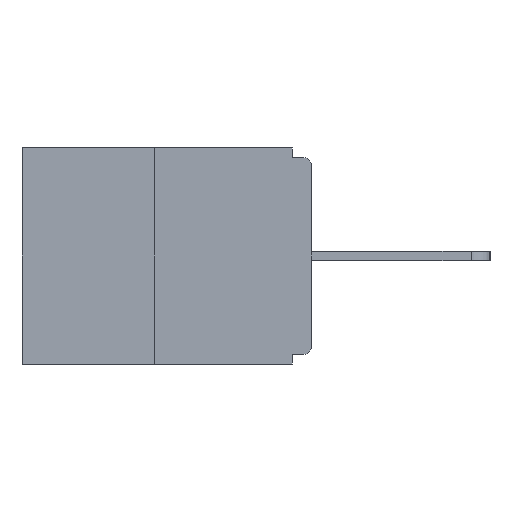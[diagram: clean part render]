
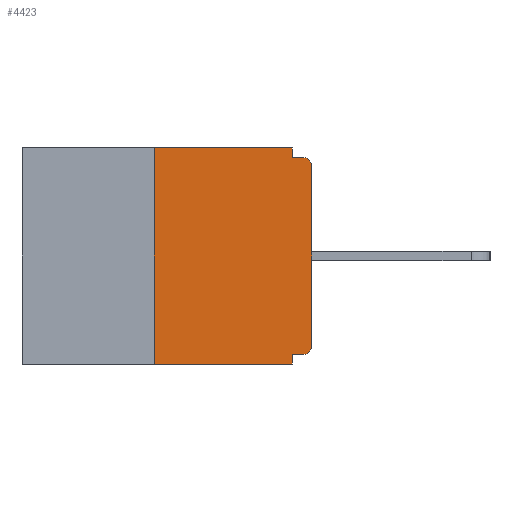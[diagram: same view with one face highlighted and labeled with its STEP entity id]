
A CAD part, left-side view. The second image highlights one B-rep face of the part: STEP entity #4423.
In plain terms, the highlighted planar face has unit normal (-1, 0, 0).
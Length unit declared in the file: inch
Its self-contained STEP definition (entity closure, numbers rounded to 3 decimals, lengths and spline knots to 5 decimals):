
#121 = VECTOR ( 'NONE', #13060, 39.37008 ) ;
#340 = DIRECTION ( 'NONE',  ( 0., -1., 0. ) ) ;
#589 = LINE ( 'NONE', #2105, #20550 ) ;
#617 = EDGE_CURVE ( 'NONE', #13745, #7215, #2869, .T. ) ;
#618 = ORIENTED_EDGE ( 'NONE', *, *, #7090, .F. ) ;
#761 = DIRECTION ( 'NONE',  ( 0., 0., -1. ) ) ;
#1275 = VECTOR ( 'NONE', #15294, 39.37008 ) ;
#1450 = CARTESIAN_POINT ( 'NONE',  ( 0., 0., -0.03 ) ) ;
#1510 = AXIS2_PLACEMENT_3D ( 'NONE', #13704, #17521, #15664 ) ;
#1878 = CARTESIAN_POINT ( 'NONE',  ( 0., 0.031, -0.015 ) ) ;
#2105 = CARTESIAN_POINT ( 'NONE',  ( 0., 0., -0.015 ) ) ;
#2442 = VERTEX_POINT ( 'NONE', #18229 ) ;
#2542 = ORIENTED_EDGE ( 'NONE', *, *, #14421, .F. ) ;
#2869 = CIRCLE ( 'NONE', #14694, 0.015 ) ;
#3036 = CARTESIAN_POINT ( 'NONE',  ( 0., 0., 0. ) ) ;
#3769 = CARTESIAN_POINT ( 'NONE',  ( 0., 0.46, 0. ) ) ;
#4001 = DIRECTION ( 'NONE',  ( 1., 0., 0. ) ) ;
#4075 = DIRECTION ( 'NONE',  ( 0., -1., 0. ) ) ;
#4110 = FACE_OUTER_BOUND ( 'NONE', #20853, .T. ) ;
#4326 = VERTEX_POINT ( 'NONE', #15697 ) ;
#4423 = ADVANCED_FACE ( 'NONE', ( #4110 ), #7456, .F. ) ;
#4606 = VERTEX_POINT ( 'NONE', #6181 ) ;
#5481 = DIRECTION ( 'NONE',  ( 0., 0., -1. ) ) ;
#5856 = ORIENTED_EDGE ( 'NONE', *, *, #6745, .F. ) ;
#5961 = CIRCLE ( 'NONE', #1510, 0.015 ) ;
#6181 = CARTESIAN_POINT ( 'NONE',  ( 0., 0.25, -0.343 ) ) ;
#6287 = EDGE_CURVE ( 'NONE', #17212, #13745, #14839, .T. ) ;
#6362 = ORIENTED_EDGE ( 'NONE', *, *, #16251, .T. ) ;
#6635 = ORIENTED_EDGE ( 'NONE', *, *, #20191, .F. ) ;
#6745 = EDGE_CURVE ( 'NONE', #4606, #4326, #9105, .T. ) ;
#6884 = AXIS2_PLACEMENT_3D ( 'NONE', #3769, #4001, #10833 ) ;
#7090 = EDGE_CURVE ( 'NONE', #10449, #21361, #14043, .T. ) ;
#7215 = VERTEX_POINT ( 'NONE', #16700 ) ;
#7456 = PLANE ( 'NONE',  #6884 ) ;
#8200 = LINE ( 'NONE', #15263, #121 ) ;
#8759 = DIRECTION ( 'NONE',  ( 0., 0., 1. ) ) ;
#9105 = LINE ( 'NONE', #19409, #10096 ) ;
#9154 = LINE ( 'NONE', #16207, #9978 ) ;
#9737 = LINE ( 'NONE', #20509, #1275 ) ;
#9885 = ORIENTED_EDGE ( 'NONE', *, *, #617, .T. ) ;
#9978 = VECTOR ( 'NONE', #340, 39.37008 ) ;
#10065 = VERTEX_POINT ( 'NONE', #20390 ) ;
#10096 = VECTOR ( 'NONE', #8759, 39.37008 ) ;
#10190 = EDGE_CURVE ( 'NONE', #17367, #10065, #9737, .T. ) ;
#10449 = VERTEX_POINT ( 'NONE', #19798 ) ;
#10833 = DIRECTION ( 'NONE',  ( 0., 0., -1. ) ) ;
#11376 = DIRECTION ( 'NONE',  ( 0., 0., 1. ) ) ;
#11889 = ORIENTED_EDGE ( 'NONE', *, *, #22378, .F. ) ;
#12240 = CARTESIAN_POINT ( 'NONE',  ( 0., 0., -0.313 ) ) ;
#12807 = ORIENTED_EDGE ( 'NONE', *, *, #6287, .T. ) ;
#13032 = CARTESIAN_POINT ( 'NONE',  ( 0., 0.015, -0.03 ) ) ;
#13060 = DIRECTION ( 'NONE',  ( 0., 0., -1. ) ) ;
#13455 = LINE ( 'NONE', #16692, #21918 ) ;
#13704 = CARTESIAN_POINT ( 'NONE',  ( 0., 0.015, -0.313 ) ) ;
#13745 = VERTEX_POINT ( 'NONE', #1450 ) ;
#14043 = LINE ( 'NONE', #22842, #20082 ) ;
#14129 = VECTOR ( 'NONE', #11376, 39.37008 ) ;
#14421 = EDGE_CURVE ( 'NONE', #4326, #10449, #9154, .T. ) ;
#14694 = AXIS2_PLACEMENT_3D ( 'NONE', #13032, #21727, #761 ) ;
#14839 = LINE ( 'NONE', #3036, #14129 ) ;
#14956 = DIRECTION ( 'NONE',  ( 0., -1., 0. ) ) ;
#15263 = CARTESIAN_POINT ( 'NONE',  ( 0., 0.031, -0.343 ) ) ;
#15294 = DIRECTION ( 'NONE',  ( 0., 1., 0. ) ) ;
#15664 = DIRECTION ( 'NONE',  ( 0., 0., -1. ) ) ;
#15697 = CARTESIAN_POINT ( 'NONE',  ( 0., 0.25, 0. ) ) ;
#16207 = CARTESIAN_POINT ( 'NONE',  ( 0., 0.46, 0. ) ) ;
#16251 = EDGE_CURVE ( 'NONE', #17367, #17212, #5961, .T. ) ;
#16692 = CARTESIAN_POINT ( 'NONE',  ( 0., 0.46, -0.343 ) ) ;
#16700 = CARTESIAN_POINT ( 'NONE',  ( 0., 0.015, -0.015 ) ) ;
#17016 = ORIENTED_EDGE ( 'NONE', *, *, #10190, .F. ) ;
#17212 = VERTEX_POINT ( 'NONE', #12240 ) ;
#17367 = VERTEX_POINT ( 'NONE', #18258 ) ;
#17521 = DIRECTION ( 'NONE',  ( -1., 0., 0. ) ) ;
#17593 = ORIENTED_EDGE ( 'NONE', *, *, #17799, .T. ) ;
#17799 = EDGE_CURVE ( 'NONE', #4606, #2442, #13455, .T. ) ;
#18229 = CARTESIAN_POINT ( 'NONE',  ( 0., 0.031, -0.343 ) ) ;
#18258 = CARTESIAN_POINT ( 'NONE',  ( 0., 0.015, -0.328 ) ) ;
#19409 = CARTESIAN_POINT ( 'NONE',  ( 0., 0.25, 0. ) ) ;
#19798 = CARTESIAN_POINT ( 'NONE',  ( 0., 0.031, 0. ) ) ;
#20082 = VECTOR ( 'NONE', #5481, 39.37008 ) ;
#20191 = EDGE_CURVE ( 'NONE', #10065, #2442, #8200, .T. ) ;
#20390 = CARTESIAN_POINT ( 'NONE',  ( 0., 0.031, -0.328 ) ) ;
#20509 = CARTESIAN_POINT ( 'NONE',  ( 0., 0., -0.328 ) ) ;
#20550 = VECTOR ( 'NONE', #4075, 39.37008 ) ;
#20853 = EDGE_LOOP ( 'NONE', ( #2542, #5856, #17593, #6635, #17016, #6362, #12807, #9885, #11889, #618 ) ) ;
#21361 = VERTEX_POINT ( 'NONE', #1878 ) ;
#21727 = DIRECTION ( 'NONE',  ( -1., 0., 0. ) ) ;
#21918 = VECTOR ( 'NONE', #14956, 39.37008 ) ;
#22378 = EDGE_CURVE ( 'NONE', #21361, #7215, #589, .T. ) ;
#22842 = CARTESIAN_POINT ( 'NONE',  ( 0., 0.031, 0. ) ) ;
